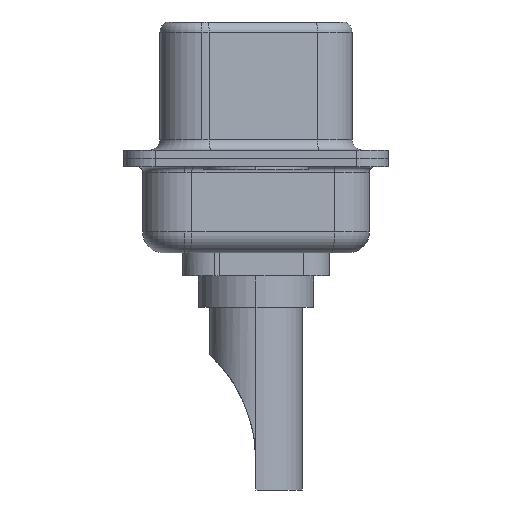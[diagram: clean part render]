
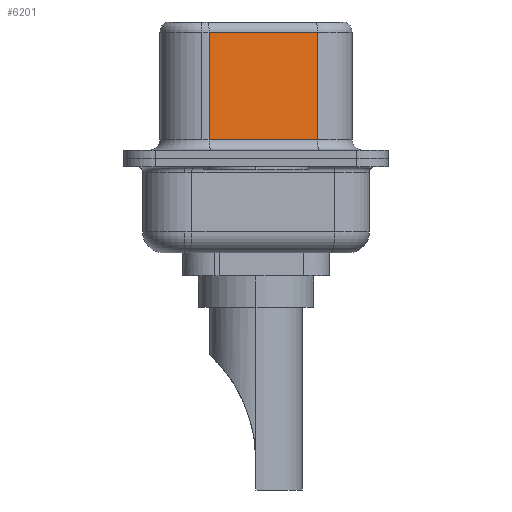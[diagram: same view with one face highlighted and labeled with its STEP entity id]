
A CAD part, left-side view. The second image highlights one B-rep face of the part: STEP entity #6201.
In plain terms, the highlighted planar face has unit normal (-0.985, -0.174, 0).
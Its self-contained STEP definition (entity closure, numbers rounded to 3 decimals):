
#877 = CARTESIAN_POINT ( 'NONE',  ( 4.565, -2.927, 6.02 ) ) ;
#1522 = EDGE_CURVE ( 'NONE', #11721, #8947, #1948, .T. ) ;
#1681 = DIRECTION ( 'NONE',  ( 0., 0., -1. ) ) ;
#1948 = LINE ( 'NONE', #877, #7773 ) ;
#1978 = CARTESIAN_POINT ( 'NONE',  ( 4.565, -2.927, 0.9 ) ) ;
#2202 = EDGE_LOOP ( 'NONE', ( #4970, #5051, #5279, #9581 ) ) ;
#2234 = AXIS2_PLACEMENT_3D ( 'NONE', #6139, #12754, #7788 ) ;
#3392 = DIRECTION ( 'NONE',  ( 0.174, -0.985, 0. ) ) ;
#3711 = DIRECTION ( 'NONE',  ( -0.174, 0.985, 0. ) ) ;
#4970 = ORIENTED_EDGE ( 'NONE', *, *, #5531, .F. ) ;
#5051 = ORIENTED_EDGE ( 'NONE', *, *, #1522, .T. ) ;
#5279 = ORIENTED_EDGE ( 'NONE', *, *, #8775, .T. ) ;
#5531 = EDGE_CURVE ( 'NONE', #11721, #10215, #6435, .T. ) ;
#5838 = LINE ( 'NONE', #6515, #8455 ) ;
#6139 = CARTESIAN_POINT ( 'NONE',  ( 4.565, -2.927, 6.52 ) ) ;
#6201 = ADVANCED_FACE ( 'NONE', ( #10406 ), #9542, .F. ) ;
#6435 = LINE ( 'NONE', #12031, #9052 ) ;
#6515 = CARTESIAN_POINT ( 'NONE',  ( 3.655, 2.233, 6.52 ) ) ;
#6901 = LINE ( 'NONE', #9609, #9187 ) ;
#7005 = EDGE_CURVE ( 'NONE', #9577, #10215, #6901, .T. ) ;
#7773 = VECTOR ( 'NONE', #3711, 1000. ) ;
#7788 = DIRECTION ( 'NONE',  ( -0.174, 0.985, 0. ) ) ;
#8063 = CARTESIAN_POINT ( 'NONE',  ( 3.655, 2.233, 6.02 ) ) ;
#8455 = VECTOR ( 'NONE', #12114, 1000. ) ;
#8775 = EDGE_CURVE ( 'NONE', #8947, #9577, #5838, .T. ) ;
#8947 = VERTEX_POINT ( 'NONE', #8063 ) ;
#9052 = VECTOR ( 'NONE', #1681, 1000. ) ;
#9187 = VECTOR ( 'NONE', #3392, 1000. ) ;
#9542 = PLANE ( 'NONE',  #2234 ) ;
#9577 = VERTEX_POINT ( 'NONE', #13806 ) ;
#9581 = ORIENTED_EDGE ( 'NONE', *, *, #7005, .T. ) ;
#9609 = CARTESIAN_POINT ( 'NONE',  ( 4.565, -2.927, 0.9 ) ) ;
#10215 = VERTEX_POINT ( 'NONE', #1978 ) ;
#10406 = FACE_OUTER_BOUND ( 'NONE', #2202, .T. ) ;
#11721 = VERTEX_POINT ( 'NONE', #11856 ) ;
#11856 = CARTESIAN_POINT ( 'NONE',  ( 4.565, -2.927, 6.02 ) ) ;
#12031 = CARTESIAN_POINT ( 'NONE',  ( 4.565, -2.927, 6.52 ) ) ;
#12114 = DIRECTION ( 'NONE',  ( 0., 0., -1. ) ) ;
#12754 = DIRECTION ( 'NONE',  ( 0.985, 0.174, 0. ) ) ;
#13806 = CARTESIAN_POINT ( 'NONE',  ( 3.655, 2.233, 0.9 ) ) ;
